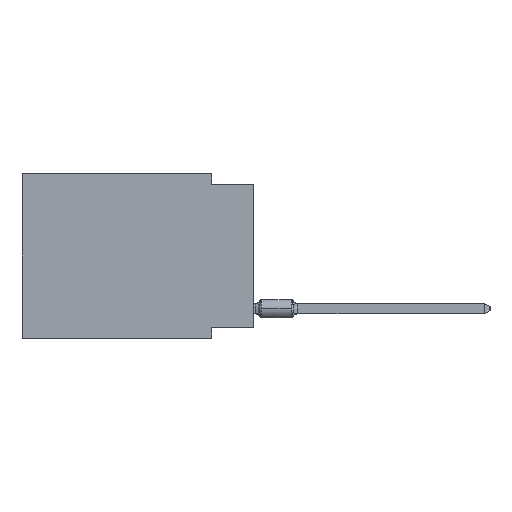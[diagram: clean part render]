
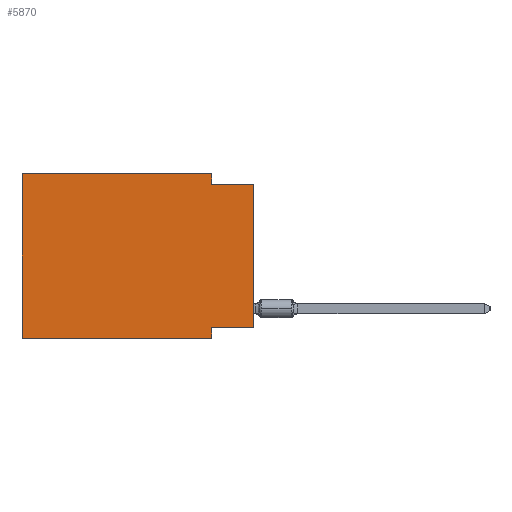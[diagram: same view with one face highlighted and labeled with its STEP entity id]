
A CAD part, left-side view. The second image highlights one B-rep face of the part: STEP entity #5870.
In plain terms, the highlighted planar face has unit normal (-1, 0, 0).
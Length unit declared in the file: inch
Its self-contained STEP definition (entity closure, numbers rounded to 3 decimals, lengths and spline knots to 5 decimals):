
#320 = DIRECTION ( 'NONE',  ( 0., 0., -1. ) ) ;
#1240 = VECTOR ( 'NONE', #23892, 39.37008 ) ;
#2153 = CARTESIAN_POINT ( 'NONE',  ( 0., 0.1, -0.39 ) ) ;
#2354 = ORIENTED_EDGE ( 'NONE', *, *, #6212, .F. ) ;
#2417 = VERTEX_POINT ( 'NONE', #29286 ) ;
#2602 = FACE_OUTER_BOUND ( 'NONE', #32809, .T. ) ;
#2991 = LINE ( 'NONE', #6202, #8275 ) ;
#3811 = DIRECTION ( 'NONE',  ( 0., 0., -1. ) ) ;
#4727 = CARTESIAN_POINT ( 'NONE',  ( 0., 0.1, -0.39 ) ) ;
#4843 = DIRECTION ( 'NONE',  ( 0., -1., 0. ) ) ;
#5514 = VERTEX_POINT ( 'NONE', #28638 ) ;
#5858 = EDGE_CURVE ( 'NONE', #2417, #9468, #17363, .T. ) ;
#5870 = ADVANCED_FACE ( 'NONE', ( #2602 ), #20029, .F. ) ;
#5997 = DIRECTION ( 'NONE',  ( 1., 0., 0. ) ) ;
#6202 = CARTESIAN_POINT ( 'NONE',  ( 0., 0., -0.365 ) ) ;
#6212 = EDGE_CURVE ( 'NONE', #12856, #15905, #25312, .T. ) ;
#7882 = LINE ( 'NONE', #24748, #7985 ) ;
#7985 = VECTOR ( 'NONE', #4843, 39.37008 ) ;
#8275 = VECTOR ( 'NONE', #31978, 39.37008 ) ;
#8434 = ORIENTED_EDGE ( 'NONE', *, *, #18481, .F. ) ;
#9468 = VERTEX_POINT ( 'NONE', #19487 ) ;
#9985 = AXIS2_PLACEMENT_3D ( 'NONE', #22685, #5997, #320 ) ;
#10198 = EDGE_CURVE ( 'NONE', #5514, #12115, #36055, .T. ) ;
#10566 = CARTESIAN_POINT ( 'NONE',  ( 0., 0.1, 0. ) ) ;
#11362 = ORIENTED_EDGE ( 'NONE', *, *, #25508, .T. ) ;
#11747 = LINE ( 'NONE', #28620, #23754 ) ;
#12115 = VERTEX_POINT ( 'NONE', #4727 ) ;
#12154 = CARTESIAN_POINT ( 'NONE',  ( 0., 0.55, 0. ) ) ;
#12713 = EDGE_CURVE ( 'NONE', #23797, #5514, #2991, .T. ) ;
#12856 = VERTEX_POINT ( 'NONE', #27410 ) ;
#13007 = VECTOR ( 'NONE', #22247, 39.37008 ) ;
#14614 = LINE ( 'NONE', #12154, #1240 ) ;
#15446 = VECTOR ( 'NONE', #3811, 39.37008 ) ;
#15548 = LINE ( 'NONE', #32607, #15446 ) ;
#15808 = ORIENTED_EDGE ( 'NONE', *, *, #12713, .F. ) ;
#15905 = VERTEX_POINT ( 'NONE', #10566 ) ;
#17363 = LINE ( 'NONE', #28919, #32959 ) ;
#18397 = ORIENTED_EDGE ( 'NONE', *, *, #20238, .T. ) ;
#18481 = EDGE_CURVE ( 'NONE', #19587, #12856, #14614, .T. ) ;
#19487 = CARTESIAN_POINT ( 'NONE',  ( 0., 0., -0.025 ) ) ;
#19587 = VERTEX_POINT ( 'NONE', #22103 ) ;
#20029 = PLANE ( 'NONE',  #9985 ) ;
#20238 = EDGE_CURVE ( 'NONE', #19587, #12115, #7882, .T. ) ;
#22103 = CARTESIAN_POINT ( 'NONE',  ( 0., 0.55, -0.39 ) ) ;
#22247 = DIRECTION ( 'NONE',  ( 0., 0., -1. ) ) ;
#22474 = CARTESIAN_POINT ( 'NONE',  ( 0., 0.55, 0. ) ) ;
#22685 = CARTESIAN_POINT ( 'NONE',  ( 0., 0.55, 0. ) ) ;
#23754 = VECTOR ( 'NONE', #29358, 39.37008 ) ;
#23797 = VERTEX_POINT ( 'NONE', #24058 ) ;
#23892 = DIRECTION ( 'NONE',  ( 0., 0., 1. ) ) ;
#24058 = CARTESIAN_POINT ( 'NONE',  ( 0., 0., -0.365 ) ) ;
#24431 = ORIENTED_EDGE ( 'NONE', *, *, #5858, .F. ) ;
#24748 = CARTESIAN_POINT ( 'NONE',  ( 0., 0.55, -0.39 ) ) ;
#24981 = VECTOR ( 'NONE', #34025, 39.37008 ) ;
#25312 = LINE ( 'NONE', #22474, #24981 ) ;
#25508 = EDGE_CURVE ( 'NONE', #23797, #9468, #11747, .T. ) ;
#26451 = DIRECTION ( 'NONE',  ( 0., -1., 0. ) ) ;
#27410 = CARTESIAN_POINT ( 'NONE',  ( 0., 0.55, 0. ) ) ;
#27895 = ORIENTED_EDGE ( 'NONE', *, *, #10198, .F. ) ;
#28620 = CARTESIAN_POINT ( 'NONE',  ( 0., 0., 0. ) ) ;
#28638 = CARTESIAN_POINT ( 'NONE',  ( 0., 0.1, -0.365 ) ) ;
#28919 = CARTESIAN_POINT ( 'NONE',  ( 0., 0., -0.025 ) ) ;
#29286 = CARTESIAN_POINT ( 'NONE',  ( 0., 0.1, -0.025 ) ) ;
#29358 = DIRECTION ( 'NONE',  ( 0., 0., 1. ) ) ;
#29920 = ORIENTED_EDGE ( 'NONE', *, *, #30637, .F. ) ;
#30637 = EDGE_CURVE ( 'NONE', #15905, #2417, #15548, .T. ) ;
#31978 = DIRECTION ( 'NONE',  ( 0., 1., 0. ) ) ;
#32607 = CARTESIAN_POINT ( 'NONE',  ( 0., 0.1, 0. ) ) ;
#32809 = EDGE_LOOP ( 'NONE', ( #11362, #24431, #29920, #2354, #8434, #18397, #27895, #15808 ) ) ;
#32959 = VECTOR ( 'NONE', #26451, 39.37008 ) ;
#34025 = DIRECTION ( 'NONE',  ( 0., -1., 0. ) ) ;
#36055 = LINE ( 'NONE', #2153, #13007 ) ;
